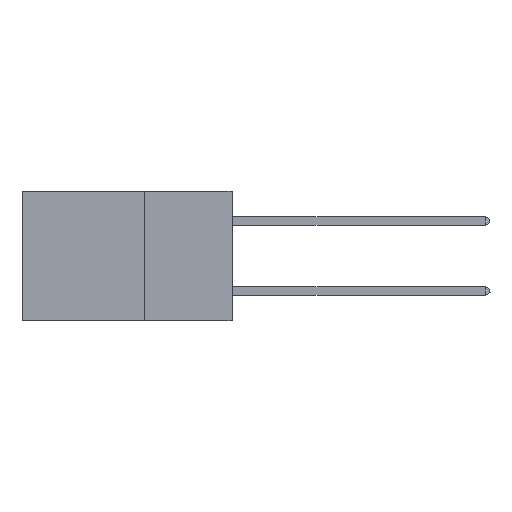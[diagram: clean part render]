
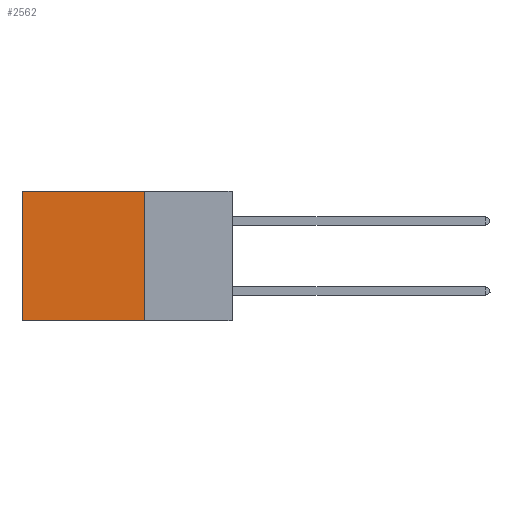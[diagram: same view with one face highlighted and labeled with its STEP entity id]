
A CAD part, left-side view. The second image highlights one B-rep face of the part: STEP entity #2562.
In plain terms, the highlighted planar face has unit normal (-1, 0, 0).
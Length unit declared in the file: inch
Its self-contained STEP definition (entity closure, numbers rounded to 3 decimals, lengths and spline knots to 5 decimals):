
#406 = VECTOR ( 'NONE', #13522, 39.37008 ) ;
#784 = VERTEX_POINT ( 'NONE', #17775 ) ;
#864 = DIRECTION ( 'NONE',  ( 0., 0., -1. ) ) ;
#1671 = EDGE_CURVE ( 'NONE', #3315, #16073, #7505, .T. ) ;
#2562 = ADVANCED_FACE ( 'NONE', ( #9339 ), #22448, .F. ) ;
#3043 = CARTESIAN_POINT ( 'NONE',  ( 0.2875, 0.25, 0. ) ) ;
#3201 = DIRECTION ( 'NONE',  ( 1., 0., 0. ) ) ;
#3315 = VERTEX_POINT ( 'NONE', #29987 ) ;
#4233 = EDGE_CURVE ( 'NONE', #3315, #5085, #28425, .T. ) ;
#4824 = VECTOR ( 'NONE', #19482, 39.37008 ) ;
#5085 = VERTEX_POINT ( 'NONE', #30233 ) ;
#5564 = LINE ( 'NONE', #21152, #4824 ) ;
#7505 = LINE ( 'NONE', #3043, #30456 ) ;
#7815 = DIRECTION ( 'NONE',  ( 0., 1., 0. ) ) ;
#9339 = FACE_OUTER_BOUND ( 'NONE', #23825, .T. ) ;
#11343 = LINE ( 'NONE', #27857, #406 ) ;
#12362 = EDGE_CURVE ( 'NONE', #16073, #784, #5564, .T. ) ;
#12843 = CARTESIAN_POINT ( 'NONE',  ( 0.2875, 0.6, 0. ) ) ;
#13522 = DIRECTION ( 'NONE',  ( 0., 1., 0. ) ) ;
#16073 = VERTEX_POINT ( 'NONE', #12843 ) ;
#16887 = ORIENTED_EDGE ( 'NONE', *, *, #4233, .F. ) ;
#17775 = CARTESIAN_POINT ( 'NONE',  ( 0.2875, 0.6, -0.37 ) ) ;
#17866 = VECTOR ( 'NONE', #24071, 39.37008 ) ;
#19482 = DIRECTION ( 'NONE',  ( 0., 0., -1. ) ) ;
#21152 = CARTESIAN_POINT ( 'NONE',  ( 0.2875, 0.6, 0. ) ) ;
#21998 = ORIENTED_EDGE ( 'NONE', *, *, #1671, .T. ) ;
#22448 = PLANE ( 'NONE',  #30940 ) ;
#23590 = EDGE_CURVE ( 'NONE', #5085, #784, #11343, .T. ) ;
#23825 = EDGE_LOOP ( 'NONE', ( #27135, #30032, #16887, #21998 ) ) ;
#24071 = DIRECTION ( 'NONE',  ( 0., 0., -1. ) ) ;
#25059 = CARTESIAN_POINT ( 'NONE',  ( 0.2875, 0.25, 0. ) ) ;
#27135 = ORIENTED_EDGE ( 'NONE', *, *, #12362, .T. ) ;
#27857 = CARTESIAN_POINT ( 'NONE',  ( 0.2875, 0.25, -0.37 ) ) ;
#28425 = LINE ( 'NONE', #28802, #17866 ) ;
#28802 = CARTESIAN_POINT ( 'NONE',  ( 0.2875, 0.25, 0. ) ) ;
#29987 = CARTESIAN_POINT ( 'NONE',  ( 0.2875, 0.25, 0. ) ) ;
#30032 = ORIENTED_EDGE ( 'NONE', *, *, #23590, .F. ) ;
#30233 = CARTESIAN_POINT ( 'NONE',  ( 0.2875, 0.25, -0.37 ) ) ;
#30456 = VECTOR ( 'NONE', #7815, 39.37008 ) ;
#30940 = AXIS2_PLACEMENT_3D ( 'NONE', #25059, #3201, #864 ) ;
